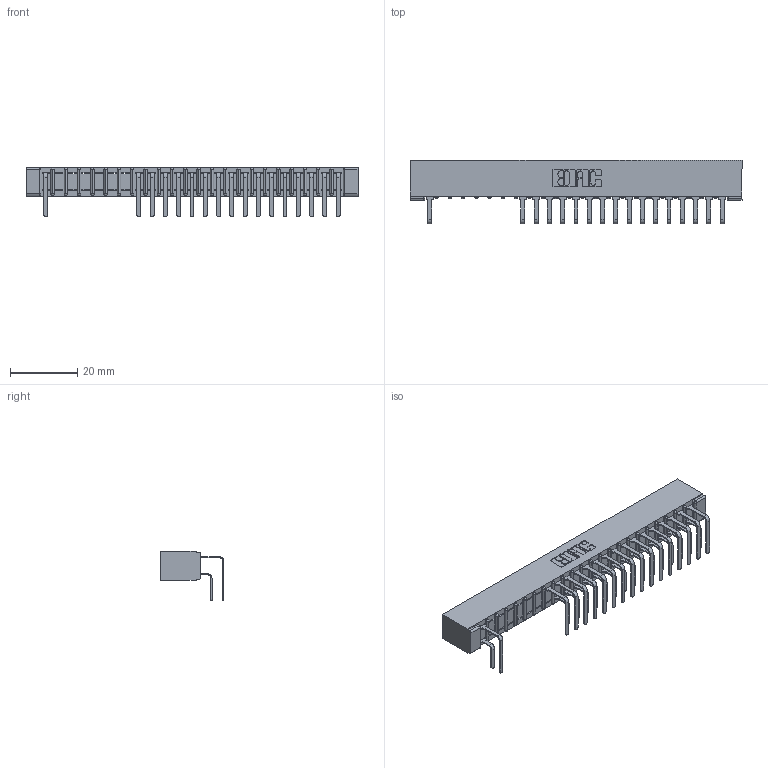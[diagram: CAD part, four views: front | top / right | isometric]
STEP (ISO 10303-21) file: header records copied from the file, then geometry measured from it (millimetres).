
FILE_DESCRIPTION (( 'STEP AP203' ), '1' );
FILE_NAME ('307-046-558-201.STEP', '2018-08-06T03:18:30', ( '' ), ( '' ), 'SwSTEP 2.0', 'SolidWorks 2016', '' );
FILE_SCHEMA (( 'CONFIG_CONTROL_DESIGN' ));
Length unit declared in the file: inch
Products named in the file (4): 307-046-558-201; 307 Part_No Mounting Lugs; 307-290-001_558 559 - 1 (Single); 307-290-001_558 - 2 (Single)
Assembly tree (34 placements, depth 2):
  307-046-558-201
    307 Part_No Mounting Lugs
    307-290-001_558 559 - 1 (Single)  x16
    307-290-001_558 - 2 (Single)  x17
Bounding box: 99.01 x 18.96 x 14.81 mm (x, y, z)
Volume: 6688.9 mm3; surface area: 12176.6 mm2
Topology: 34 solids, 34 shells, 1914 faces, 5401 edges, 3490 vertices
Faces by surface type: plane 1233, cylinder 633, sphere 48
Entity records: 23549 total; most frequent: CARTESIAN_POINT 3912, ORIENTED_EDGE 3886, DIRECTION 3825, EDGE_CURVE 1943, VECTOR 1483, LINE 1483, VERTEX_POINT 1258, AXIS2_PLACEMENT_3D 1171
